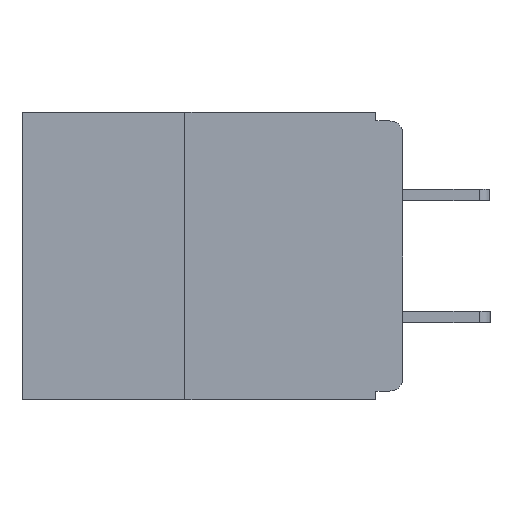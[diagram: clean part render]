
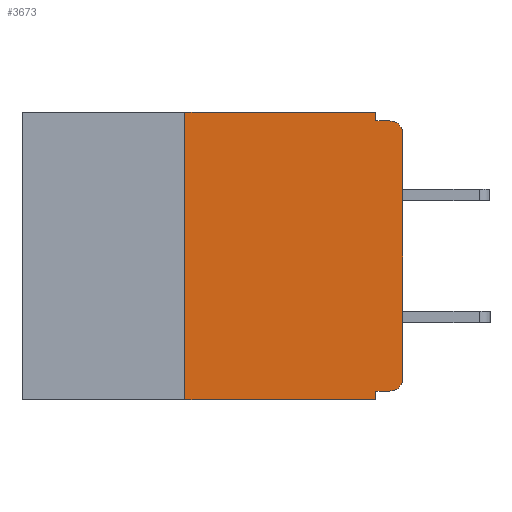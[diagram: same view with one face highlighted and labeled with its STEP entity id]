
A CAD part, left-side view. The second image highlights one B-rep face of the part: STEP entity #3673.
In plain terms, the highlighted planar face has unit normal (-1, 0, 0).
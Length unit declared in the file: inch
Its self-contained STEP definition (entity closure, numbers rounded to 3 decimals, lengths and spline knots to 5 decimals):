
#214 = VERTEX_POINT ( 'NONE', #3975 ) ;
#220 = CARTESIAN_POINT ( 'NONE',  ( 0., 0.015, -0.01 ) ) ;
#228 = VECTOR ( 'NONE', #14851, 39.37008 ) ;
#659 = EDGE_CURVE ( 'NONE', #20680, #16662, #14905, .T. ) ;
#1102 = VECTOR ( 'NONE', #8023, 39.37008 ) ;
#1373 = VERTEX_POINT ( 'NONE', #12203 ) ;
#1493 = CARTESIAN_POINT ( 'NONE',  ( 0., 0.437, -0.33 ) ) ;
#1752 = AXIS2_PLACEMENT_3D ( 'NONE', #20564, #20383, #16666 ) ;
#2087 = CARTESIAN_POINT ( 'NONE',  ( 0., 0.25, -0.33 ) ) ;
#3480 = LINE ( 'NONE', #5053, #6239 ) ;
#3517 = VECTOR ( 'NONE', #8570, 39.37008 ) ;
#3660 = CARTESIAN_POINT ( 'NONE',  ( 0., 0.031, 0. ) ) ;
#3673 = ADVANCED_FACE ( 'NONE', ( #9517 ), #16456, .F. ) ;
#3975 = CARTESIAN_POINT ( 'NONE',  ( 0., 0.031, -0.32 ) ) ;
#4042 = VERTEX_POINT ( 'NONE', #3660 ) ;
#4180 = DIRECTION ( 'NONE',  ( 0., 0., 1. ) ) ;
#4327 = DIRECTION ( 'NONE',  ( 0., 0., -1. ) ) ;
#4402 = CARTESIAN_POINT ( 'NONE',  ( 0., 0.437, 0. ) ) ;
#4429 = DIRECTION ( 'NONE',  ( -1., 0., 0. ) ) ;
#4447 = CARTESIAN_POINT ( 'NONE',  ( 0., 0.015, -0.305 ) ) ;
#4482 = CARTESIAN_POINT ( 'NONE',  ( 0., 0., 0. ) ) ;
#4957 = CARTESIAN_POINT ( 'NONE',  ( 0., 0., -0.32 ) ) ;
#5051 = CIRCLE ( 'NONE', #15504, 0.015 ) ;
#5053 = CARTESIAN_POINT ( 'NONE',  ( 0., 0.031, -0.33 ) ) ;
#5128 = DIRECTION ( 'NONE',  ( 0., 0., -1. ) ) ;
#5815 = DIRECTION ( 'NONE',  ( 0., 0., -1. ) ) ;
#5828 = DIRECTION ( 'NONE',  ( -1., 0., 0. ) ) ;
#5885 = CARTESIAN_POINT ( 'NONE',  ( 0., 0.015, -0.025 ) ) ;
#6052 = EDGE_CURVE ( 'NONE', #19906, #6797, #5051, .T. ) ;
#6065 = ORIENTED_EDGE ( 'NONE', *, *, #9235, .T. ) ;
#6172 = EDGE_CURVE ( 'NONE', #18469, #14386, #19288, .T. ) ;
#6239 = VECTOR ( 'NONE', #5128, 39.37008 ) ;
#6605 = VECTOR ( 'NONE', #8711, 39.37008 ) ;
#6797 = VERTEX_POINT ( 'NONE', #220 ) ;
#6887 = CARTESIAN_POINT ( 'NONE',  ( 0., 0., -0.01 ) ) ;
#7294 = EDGE_CURVE ( 'NONE', #4042, #12562, #18018, .T. ) ;
#7601 = ORIENTED_EDGE ( 'NONE', *, *, #6052, .T. ) ;
#8010 = ORIENTED_EDGE ( 'NONE', *, *, #21052, .F. ) ;
#8023 = DIRECTION ( 'NONE',  ( 0., 0., -1. ) ) ;
#8542 = LINE ( 'NONE', #4957, #228 ) ;
#8570 = DIRECTION ( 'NONE',  ( 0., -1., 0. ) ) ;
#8684 = ORIENTED_EDGE ( 'NONE', *, *, #7294, .F. ) ;
#8691 = CARTESIAN_POINT ( 'NONE',  ( 0., 0.25, -0.33 ) ) ;
#8711 = DIRECTION ( 'NONE',  ( 0., 0., 1. ) ) ;
#9005 = ORIENTED_EDGE ( 'NONE', *, *, #11521, .F. ) ;
#9113 = ORIENTED_EDGE ( 'NONE', *, *, #659, .F. ) ;
#9235 = EDGE_CURVE ( 'NONE', #14386, #19906, #18908, .T. ) ;
#9287 = ORIENTED_EDGE ( 'NONE', *, *, #18637, .T. ) ;
#9517 = FACE_OUTER_BOUND ( 'NONE', #19004, .T. ) ;
#9830 = CARTESIAN_POINT ( 'NONE',  ( 0., 0., -0.025 ) ) ;
#9896 = ORIENTED_EDGE ( 'NONE', *, *, #13302, .F. ) ;
#10264 = VECTOR ( 'NONE', #17891, 39.37008 ) ;
#10643 = ORIENTED_EDGE ( 'NONE', *, *, #13867, .F. ) ;
#11264 = LINE ( 'NONE', #4402, #19295 ) ;
#11521 = EDGE_CURVE ( 'NONE', #16662, #4042, #11264, .T. ) ;
#11913 = ORIENTED_EDGE ( 'NONE', *, *, #6172, .T. ) ;
#12203 = CARTESIAN_POINT ( 'NONE',  ( 0., 0.031, -0.33 ) ) ;
#12277 = LINE ( 'NONE', #6887, #3517 ) ;
#12562 = VERTEX_POINT ( 'NONE', #16311 ) ;
#12634 = DIRECTION ( 'NONE',  ( 0., -1., 0. ) ) ;
#12660 = CARTESIAN_POINT ( 'NONE',  ( 0., 0.015, -0.32 ) ) ;
#13302 = EDGE_CURVE ( 'NONE', #214, #1373, #3480, .T. ) ;
#13867 = EDGE_CURVE ( 'NONE', #18469, #214, #8542, .T. ) ;
#14034 = CARTESIAN_POINT ( 'NONE',  ( 0., 0.031, 0. ) ) ;
#14386 = VERTEX_POINT ( 'NONE', #19220 ) ;
#14631 = LINE ( 'NONE', #1493, #10264 ) ;
#14719 = VECTOR ( 'NONE', #4180, 39.37008 ) ;
#14851 = DIRECTION ( 'NONE',  ( 0., 1., 0. ) ) ;
#14905 = LINE ( 'NONE', #8691, #6605 ) ;
#15504 = AXIS2_PLACEMENT_3D ( 'NONE', #5885, #5828, #5815 ) ;
#16111 = CARTESIAN_POINT ( 'NONE',  ( 0., 0.25, 0. ) ) ;
#16311 = CARTESIAN_POINT ( 'NONE',  ( 0., 0.031, -0.01 ) ) ;
#16456 = PLANE ( 'NONE',  #1752 ) ;
#16560 = AXIS2_PLACEMENT_3D ( 'NONE', #4447, #4429, #4327 ) ;
#16662 = VERTEX_POINT ( 'NONE', #16111 ) ;
#16666 = DIRECTION ( 'NONE',  ( 0., 0., -1. ) ) ;
#17891 = DIRECTION ( 'NONE',  ( 0., -1., 0. ) ) ;
#18018 = LINE ( 'NONE', #14034, #1102 ) ;
#18469 = VERTEX_POINT ( 'NONE', #12660 ) ;
#18637 = EDGE_CURVE ( 'NONE', #20680, #1373, #14631, .T. ) ;
#18908 = LINE ( 'NONE', #4482, #14719 ) ;
#19004 = EDGE_LOOP ( 'NONE', ( #6065, #7601, #8010, #8684, #9005, #9113, #9287, #9896, #10643, #11913 ) ) ;
#19220 = CARTESIAN_POINT ( 'NONE',  ( 0., 0., -0.305 ) ) ;
#19288 = CIRCLE ( 'NONE', #16560, 0.015 ) ;
#19295 = VECTOR ( 'NONE', #12634, 39.37008 ) ;
#19906 = VERTEX_POINT ( 'NONE', #9830 ) ;
#20383 = DIRECTION ( 'NONE',  ( 1., 0., 0. ) ) ;
#20564 = CARTESIAN_POINT ( 'NONE',  ( 0., 0.437, 0. ) ) ;
#20680 = VERTEX_POINT ( 'NONE', #2087 ) ;
#21052 = EDGE_CURVE ( 'NONE', #12562, #6797, #12277, .T. ) ;
